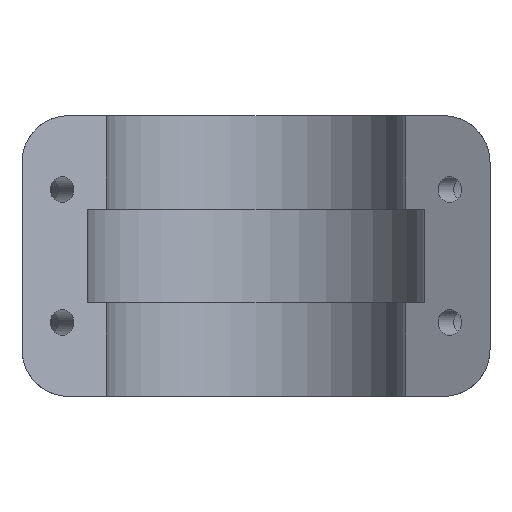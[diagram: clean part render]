
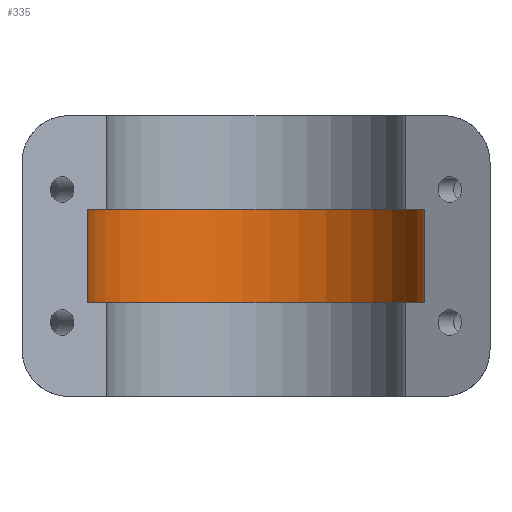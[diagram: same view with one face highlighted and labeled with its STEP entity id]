
A CAD part, left-side view. The second image highlights one B-rep face of the part: STEP entity #335.
In plain terms, the highlighted cylindrical face has radius 22.86 mm (diameter 45.72 mm), a partial arc.
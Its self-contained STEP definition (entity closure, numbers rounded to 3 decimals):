
#62 = EDGE_CURVE ( 'NONE', #941, #387, #814, .T. ) ;
#70 = EDGE_CURVE ( 'NONE', #510, #1084, #803, .T. ) ;
#153 = DIRECTION ( 'NONE',  ( 0., 0., 1. ) ) ;
#193 = CARTESIAN_POINT ( 'NONE',  ( -1.17, -22.83, 0. ) ) ;
#292 = CARTESIAN_POINT ( 'NONE',  ( 0., 0., -12.7 ) ) ;
#320 = EDGE_CURVE ( 'NONE', #387, #1084, #669, .T. ) ;
#335 = ADVANCED_FACE ( 'NONE', ( #658 ), #640, .F. ) ;
#376 = DIRECTION ( 'NONE',  ( 0., 0., 1. ) ) ;
#387 = VERTEX_POINT ( 'NONE', #537 ) ;
#510 = VERTEX_POINT ( 'NONE', #1040 ) ;
#527 = CARTESIAN_POINT ( 'NONE',  ( -1.17, -22.83, -12.7 ) ) ;
#537 = CARTESIAN_POINT ( 'NONE',  ( -1.17, -22.83, -12.7 ) ) ;
#558 = ORIENTED_EDGE ( 'NONE', *, *, #682, .F. ) ;
#594 = ORIENTED_EDGE ( 'NONE', *, *, #62, .T. ) ;
#601 = VECTOR ( 'NONE', #376, 1000. ) ;
#604 = LINE ( 'NONE', #972, #601 ) ;
#640 = CYLINDRICAL_SURFACE ( 'NONE', #1022, 22.86 ) ;
#643 = DIRECTION ( 'NONE',  ( 1., 0., 0. ) ) ;
#656 = VECTOR ( 'NONE', #153, 1000. ) ;
#657 = CARTESIAN_POINT ( 'NONE',  ( 0., 0., 0. ) ) ;
#658 = FACE_OUTER_BOUND ( 'NONE', #986, .T. ) ;
#667 = DIRECTION ( 'NONE',  ( 0., 0., -1. ) ) ;
#669 = LINE ( 'NONE', #527, #656 ) ;
#674 = DIRECTION ( 'NONE',  ( -1., 0., 0. ) ) ;
#682 = EDGE_CURVE ( 'NONE', #941, #510, #604, .T. ) ;
#710 = ORIENTED_EDGE ( 'NONE', *, *, #70, .F. ) ;
#743 = DIRECTION ( 'NONE',  ( 0., 0., 1. ) ) ;
#764 = DIRECTION ( 'NONE',  ( -1., 0., 0. ) ) ;
#778 = DIRECTION ( 'NONE',  ( 0., 0., -1. ) ) ;
#803 = CIRCLE ( 'NONE', #1141, 22.86 ) ;
#814 = CIRCLE ( 'NONE', #1007, 22.86 ) ;
#854 = ORIENTED_EDGE ( 'NONE', *, *, #320, .T. ) ;
#861 = CARTESIAN_POINT ( 'NONE',  ( 0., 0., -12.7 ) ) ;
#941 = VERTEX_POINT ( 'NONE', #1000 ) ;
#972 = CARTESIAN_POINT ( 'NONE',  ( -1.17, 22.83, -12.7 ) ) ;
#986 = EDGE_LOOP ( 'NONE', ( #558, #594, #854, #710 ) ) ;
#1000 = CARTESIAN_POINT ( 'NONE',  ( -1.17, 22.83, -12.7 ) ) ;
#1007 = AXIS2_PLACEMENT_3D ( 'NONE', #861, #778, #764 ) ;
#1022 = AXIS2_PLACEMENT_3D ( 'NONE', #292, #743, #643 ) ;
#1040 = CARTESIAN_POINT ( 'NONE',  ( -1.17, 22.83, 0. ) ) ;
#1084 = VERTEX_POINT ( 'NONE', #193 ) ;
#1141 = AXIS2_PLACEMENT_3D ( 'NONE', #657, #667, #674 ) ;
